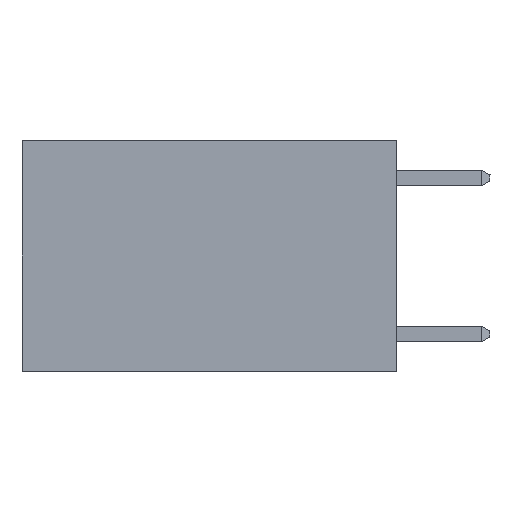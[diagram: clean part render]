
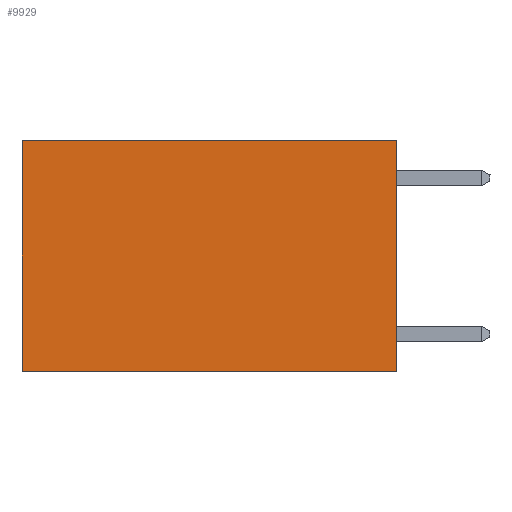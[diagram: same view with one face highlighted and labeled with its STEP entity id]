
A CAD part, left-side view. The second image highlights one B-rep face of the part: STEP entity #9929.
In plain terms, the highlighted planar face has unit normal (-1, 0, 0).
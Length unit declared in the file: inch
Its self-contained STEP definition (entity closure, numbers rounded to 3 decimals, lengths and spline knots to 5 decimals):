
#439 = ORIENTED_EDGE ( 'NONE', *, *, #9783, .F. ) ;
#745 = CARTESIAN_POINT ( 'NONE',  ( 0.2625, 0., -0.37 ) ) ;
#1237 = LINE ( 'NONE', #745, #14376 ) ;
#1369 = CARTESIAN_POINT ( 'NONE',  ( 0.2625, 0.6, -0.37 ) ) ;
#3009 = VERTEX_POINT ( 'NONE', #1369 ) ;
#3743 = CARTESIAN_POINT ( 'NONE',  ( 0.2625, 0., 0. ) ) ;
#4766 = DIRECTION ( 'NONE',  ( 0., 0., -1. ) ) ;
#5179 = LINE ( 'NONE', #3743, #5343 ) ;
#5343 = VECTOR ( 'NONE', #11114, 39.37008 ) ;
#5446 = ORIENTED_EDGE ( 'NONE', *, *, #14315, .T. ) ;
#6008 = DIRECTION ( 'NONE',  ( 0., 0., -1. ) ) ;
#8679 = VERTEX_POINT ( 'NONE', #16783 ) ;
#9661 = EDGE_LOOP ( 'NONE', ( #5446, #11880, #439, #17923 ) ) ;
#9685 = CARTESIAN_POINT ( 'NONE',  ( 0.2625, 0., 0. ) ) ;
#9783 = EDGE_CURVE ( 'NONE', #16906, #10231, #13577, .T. ) ;
#9929 = ADVANCED_FACE ( 'NONE', ( #14433 ), #18870, .F. ) ;
#10231 = VERTEX_POINT ( 'NONE', #13624 ) ;
#10904 = LINE ( 'NONE', #17047, #19590 ) ;
#11087 = EDGE_CURVE ( 'NONE', #16906, #8679, #5179, .T. ) ;
#11114 = DIRECTION ( 'NONE',  ( 0., 1., 0. ) ) ;
#11573 = DIRECTION ( 'NONE',  ( 0., 1., 0. ) ) ;
#11880 = ORIENTED_EDGE ( 'NONE', *, *, #12168, .F. ) ;
#12168 = EDGE_CURVE ( 'NONE', #10231, #3009, #1237, .T. ) ;
#12620 = DIRECTION ( 'NONE',  ( 0., 0., -1. ) ) ;
#13577 = LINE ( 'NONE', #19712, #14947 ) ;
#13624 = CARTESIAN_POINT ( 'NONE',  ( 0.2625, 0., -0.37 ) ) ;
#14242 = DIRECTION ( 'NONE',  ( 1., 0., 0. ) ) ;
#14315 = EDGE_CURVE ( 'NONE', #8679, #3009, #10904, .T. ) ;
#14376 = VECTOR ( 'NONE', #11573, 39.37008 ) ;
#14433 = FACE_OUTER_BOUND ( 'NONE', #9661, .T. ) ;
#14947 = VECTOR ( 'NONE', #6008, 39.37008 ) ;
#16783 = CARTESIAN_POINT ( 'NONE',  ( 0.2625, 0.6, 0. ) ) ;
#16906 = VERTEX_POINT ( 'NONE', #19512 ) ;
#17047 = CARTESIAN_POINT ( 'NONE',  ( 0.2625, 0.6, 0. ) ) ;
#17923 = ORIENTED_EDGE ( 'NONE', *, *, #11087, .T. ) ;
#18481 = AXIS2_PLACEMENT_3D ( 'NONE', #9685, #14242, #4766 ) ;
#18870 = PLANE ( 'NONE',  #18481 ) ;
#19512 = CARTESIAN_POINT ( 'NONE',  ( 0.2625, 0., 0. ) ) ;
#19590 = VECTOR ( 'NONE', #12620, 39.37008 ) ;
#19712 = CARTESIAN_POINT ( 'NONE',  ( 0.2625, 0., 0. ) ) ;
